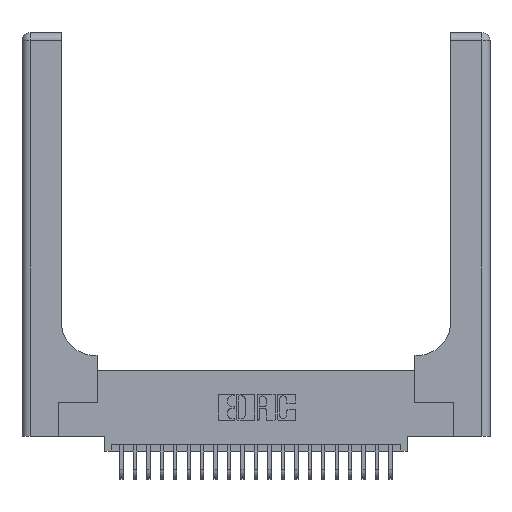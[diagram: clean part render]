
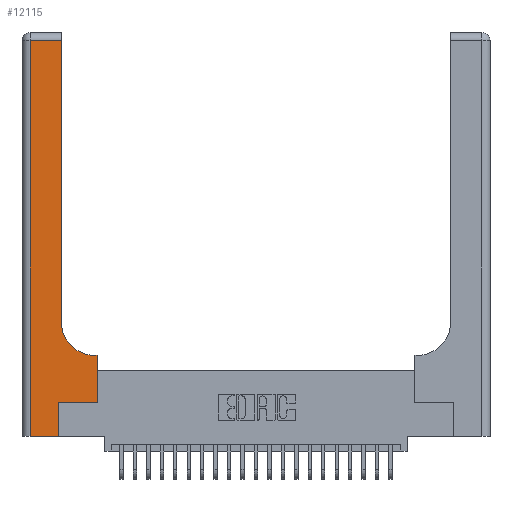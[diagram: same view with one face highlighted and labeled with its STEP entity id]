
A CAD part, top view. The second image highlights one B-rep face of the part: STEP entity #12115.
In plain terms, the highlighted planar face has unit normal (0, 0, 1).
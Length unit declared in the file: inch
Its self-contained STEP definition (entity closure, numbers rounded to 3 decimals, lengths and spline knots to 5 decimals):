
#370 = ORIENTED_EDGE ( 'NONE', *, *, #12683, .T. ) ;
#799 = VECTOR ( 'NONE', #12016, 39.37008 ) ;
#1329 = DIRECTION ( 'NONE',  ( 0., 1., 0. ) ) ;
#1400 = CARTESIAN_POINT ( 'NONE',  ( 0.5585, 0.6, 0.37 ) ) ;
#1690 = CARTESIAN_POINT ( 'NONE',  ( 0.06, 3., 0.37 ) ) ;
#1989 = EDGE_CURVE ( 'NONE', #14943, #19487, #8043, .T. ) ;
#2333 = VERTEX_POINT ( 'NONE', #17179 ) ;
#2918 = VECTOR ( 'NONE', #12745, 39.37008 ) ;
#3337 = CARTESIAN_POINT ( 'NONE',  ( 0.2915, 3., 0.37 ) ) ;
#3574 = CIRCLE ( 'NONE', #17999, 0.25 ) ;
#4135 = CARTESIAN_POINT ( 'NONE',  ( 0.5415, 0.85, 0.37 ) ) ;
#4219 = ORIENTED_EDGE ( 'NONE', *, *, #1989, .T. ) ;
#5439 = LINE ( 'NONE', #11479, #23557 ) ;
#5794 = CARTESIAN_POINT ( 'NONE',  ( 0.2915, 0.6, 0.37 ) ) ;
#6107 = EDGE_CURVE ( 'NONE', #17232, #2333, #12892, .T. ) ;
#6698 = CARTESIAN_POINT ( 'NONE',  ( 0., 2.94, 0.37 ) ) ;
#8043 = LINE ( 'NONE', #3337, #20112 ) ;
#8267 = CARTESIAN_POINT ( 'NONE',  ( 0.269, 0.25, 0.37 ) ) ;
#8569 = DIRECTION ( 'NONE',  ( 0., 0., -1. ) ) ;
#8576 = LINE ( 'NONE', #5794, #25742 ) ;
#8737 = ORIENTED_EDGE ( 'NONE', *, *, #12739, .T. ) ;
#8778 = CARTESIAN_POINT ( 'NONE',  ( 0.2915, 2.94, 0.37 ) ) ;
#8859 = CARTESIAN_POINT ( 'NONE',  ( 0.2915, 0.85, 0.37 ) ) ;
#9318 = CARTESIAN_POINT ( 'NONE',  ( 0., 0., 0.37 ) ) ;
#9855 = EDGE_CURVE ( 'NONE', #19545, #17170, #22025, .T. ) ;
#10137 = LINE ( 'NONE', #21954, #24099 ) ;
#10151 = EDGE_CURVE ( 'NONE', #16508, #14943, #3574, .T. ) ;
#10210 = EDGE_CURVE ( 'NONE', #19487, #11367, #13728, .T. ) ;
#11006 = CARTESIAN_POINT ( 'NONE',  ( 0.269, 0., 0.37 ) ) ;
#11137 = EDGE_CURVE ( 'NONE', #13554, #16508, #8576, .T. ) ;
#11153 = ORIENTED_EDGE ( 'NONE', *, *, #16647, .T. ) ;
#11282 = CARTESIAN_POINT ( 'NONE',  ( 0.06, 2.94, 0.37 ) ) ;
#11367 = VERTEX_POINT ( 'NONE', #11282 ) ;
#11479 = CARTESIAN_POINT ( 'NONE',  ( 0.269, 0., 0.37 ) ) ;
#11691 = ORIENTED_EDGE ( 'NONE', *, *, #9855, .T. ) ;
#12016 = DIRECTION ( 'NONE',  ( 1., 0., 0. ) ) ;
#12115 = ADVANCED_FACE ( 'NONE', ( #12682 ), #12487, .F. ) ;
#12487 = PLANE ( 'NONE',  #16188 ) ;
#12658 = DIRECTION ( 'NONE',  ( -1., 0., 0. ) ) ;
#12682 = FACE_OUTER_BOUND ( 'NONE', #17260, .T. ) ;
#12683 = EDGE_CURVE ( 'NONE', #2333, #13554, #10137, .T. ) ;
#12739 = EDGE_CURVE ( 'NONE', #11367, #19545, #23466, .T. ) ;
#12745 = DIRECTION ( 'NONE',  ( -1., 0., 0. ) ) ;
#12751 = ORIENTED_EDGE ( 'NONE', *, *, #11137, .T. ) ;
#12892 = LINE ( 'NONE', #8267, #799 ) ;
#13554 = VERTEX_POINT ( 'NONE', #1400 ) ;
#13728 = LINE ( 'NONE', #6698, #2918 ) ;
#14943 = VERTEX_POINT ( 'NONE', #8859 ) ;
#15811 = CARTESIAN_POINT ( 'NONE',  ( 0.269, 0.25, 0.37 ) ) ;
#16188 = AXIS2_PLACEMENT_3D ( 'NONE', #20458, #24816, #12658 ) ;
#16508 = VERTEX_POINT ( 'NONE', #21047 ) ;
#16647 = EDGE_CURVE ( 'NONE', #17170, #17232, #5439, .T. ) ;
#17170 = VERTEX_POINT ( 'NONE', #11006 ) ;
#17179 = CARTESIAN_POINT ( 'NONE',  ( 0.5585, 0.25, 0.37 ) ) ;
#17232 = VERTEX_POINT ( 'NONE', #15811 ) ;
#17260 = EDGE_LOOP ( 'NONE', ( #4219, #20030, #8737, #11691, #11153, #17708, #370, #12751, #23103 ) ) ;
#17708 = ORIENTED_EDGE ( 'NONE', *, *, #6107, .T. ) ;
#17959 = DIRECTION ( 'NONE',  ( 0., 1., 0. ) ) ;
#17999 = AXIS2_PLACEMENT_3D ( 'NONE', #4135, #8569, #22766 ) ;
#18196 = VECTOR ( 'NONE', #21179, 39.37008 ) ;
#19487 = VERTEX_POINT ( 'NONE', #8778 ) ;
#19545 = VERTEX_POINT ( 'NONE', #23060 ) ;
#19797 = DIRECTION ( 'NONE',  ( 0., -1., 0. ) ) ;
#20030 = ORIENTED_EDGE ( 'NONE', *, *, #10210, .T. ) ;
#20112 = VECTOR ( 'NONE', #21544, 39.37008 ) ;
#20458 = CARTESIAN_POINT ( 'NONE',  ( 0., 3., 0.37 ) ) ;
#21047 = CARTESIAN_POINT ( 'NONE',  ( 0.5415, 0.6, 0.37 ) ) ;
#21179 = DIRECTION ( 'NONE',  ( 1., 0., 0. ) ) ;
#21544 = DIRECTION ( 'NONE',  ( 0., 1., 0. ) ) ;
#21954 = CARTESIAN_POINT ( 'NONE',  ( 0.5585, 0.25, 0.37 ) ) ;
#22025 = LINE ( 'NONE', #9318, #18196 ) ;
#22766 = DIRECTION ( 'NONE',  ( 1., 0., 0. ) ) ;
#23060 = CARTESIAN_POINT ( 'NONE',  ( 0.06, 0., 0.37 ) ) ;
#23103 = ORIENTED_EDGE ( 'NONE', *, *, #10151, .T. ) ;
#23131 = VECTOR ( 'NONE', #19797, 39.37008 ) ;
#23466 = LINE ( 'NONE', #1690, #23131 ) ;
#23557 = VECTOR ( 'NONE', #1329, 39.37008 ) ;
#24099 = VECTOR ( 'NONE', #17959, 39.37008 ) ;
#24816 = DIRECTION ( 'NONE',  ( 0., 0., -1. ) ) ;
#25320 = DIRECTION ( 'NONE',  ( -1., 0., 0. ) ) ;
#25742 = VECTOR ( 'NONE', #25320, 39.37008 ) ;
